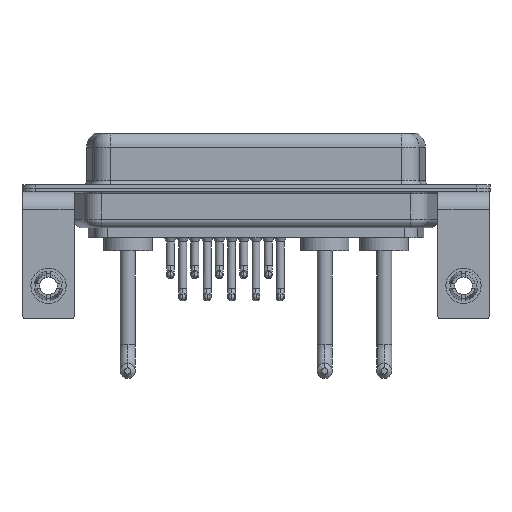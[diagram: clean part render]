
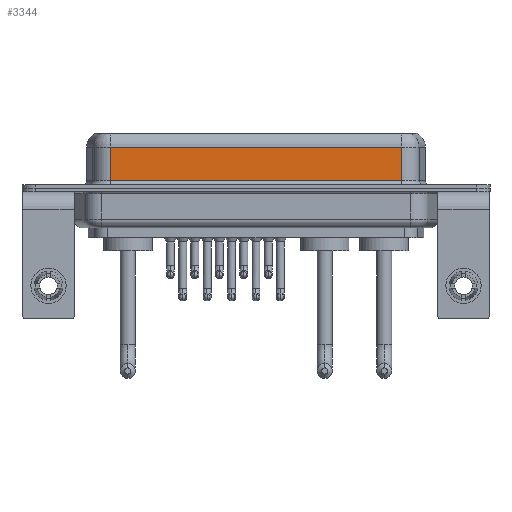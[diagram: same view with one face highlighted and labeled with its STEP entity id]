
A CAD part, front view. The second image highlights one B-rep face of the part: STEP entity #3344.
In plain terms, the highlighted planar face has unit normal (0, -1, 0).
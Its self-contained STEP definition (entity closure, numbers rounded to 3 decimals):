
#14 = VERTEX_POINT ( 'NONE', #6619 ) ;
#293 = EDGE_CURVE ( 'NONE', #15048, #534, #6072, .T. ) ;
#534 = VERTEX_POINT ( 'NONE', #2472 ) ;
#904 = PLANE ( 'NONE',  #2381 ) ;
#1193 = CARTESIAN_POINT ( 'NONE',  ( 7.013, -3.95, 6.4 ) ) ;
#1748 = VECTOR ( 'NONE', #19266, 1000. ) ;
#2381 = AXIS2_PLACEMENT_3D ( 'NONE', #7529, #20742, #5890 ) ;
#2472 = CARTESIAN_POINT ( 'NONE',  ( 40.037, -3.95, 0.9 ) ) ;
#3344 = ADVANCED_FACE ( 'NONE', ( #15761 ), #904, .F. ) ;
#5890 = DIRECTION ( 'NONE',  ( 0., 0., 1. ) ) ;
#6072 = LINE ( 'NONE', #6276, #15356 ) ;
#6276 = CARTESIAN_POINT ( 'NONE',  ( 40.037, -3.95, 0.9 ) ) ;
#6619 = CARTESIAN_POINT ( 'NONE',  ( 7.013, -3.95, 4.65 ) ) ;
#6877 = VECTOR ( 'NONE', #14435, 1000. ) ;
#7529 = CARTESIAN_POINT ( 'NONE',  ( 40.037, -3.95, 6.4 ) ) ;
#7537 = ORIENTED_EDGE ( 'NONE', *, *, #293, .T. ) ;
#7684 = LINE ( 'NONE', #9629, #1748 ) ;
#8266 = VERTEX_POINT ( 'NONE', #9728 ) ;
#8906 = DIRECTION ( 'NONE',  ( -1., 0., 0. ) ) ;
#9629 = CARTESIAN_POINT ( 'NONE',  ( 40.037, -3.95, 6.4 ) ) ;
#9728 = CARTESIAN_POINT ( 'NONE',  ( 40.037, -3.95, 4.65 ) ) ;
#10309 = LINE ( 'NONE', #17030, #17737 ) ;
#10989 = ORIENTED_EDGE ( 'NONE', *, *, #12726, .T. ) ;
#11175 = DIRECTION ( 'NONE',  ( 1., 0., 0. ) ) ;
#12726 = EDGE_CURVE ( 'NONE', #14, #15048, #16049, .T. ) ;
#13765 = ORIENTED_EDGE ( 'NONE', *, *, #14472, .F. ) ;
#14435 = DIRECTION ( 'NONE',  ( 0., 0., -1. ) ) ;
#14472 = EDGE_CURVE ( 'NONE', #8266, #534, #7684, .T. ) ;
#14817 = EDGE_LOOP ( 'NONE', ( #13765, #17876, #10989, #7537 ) ) ;
#15048 = VERTEX_POINT ( 'NONE', #20383 ) ;
#15356 = VECTOR ( 'NONE', #11175, 1000. ) ;
#15761 = FACE_OUTER_BOUND ( 'NONE', #14817, .T. ) ;
#16049 = LINE ( 'NONE', #1193, #6877 ) ;
#17030 = CARTESIAN_POINT ( 'NONE',  ( 40.037, -3.95, 4.65 ) ) ;
#17737 = VECTOR ( 'NONE', #8906, 1000. ) ;
#17876 = ORIENTED_EDGE ( 'NONE', *, *, #18522, .T. ) ;
#18522 = EDGE_CURVE ( 'NONE', #8266, #14, #10309, .T. ) ;
#19266 = DIRECTION ( 'NONE',  ( 0., 0., -1. ) ) ;
#20383 = CARTESIAN_POINT ( 'NONE',  ( 7.013, -3.95, 0.9 ) ) ;
#20742 = DIRECTION ( 'NONE',  ( 0., 1., 0. ) ) ;
